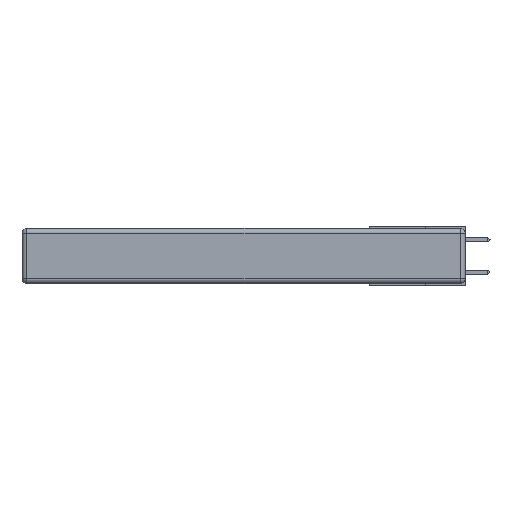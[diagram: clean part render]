
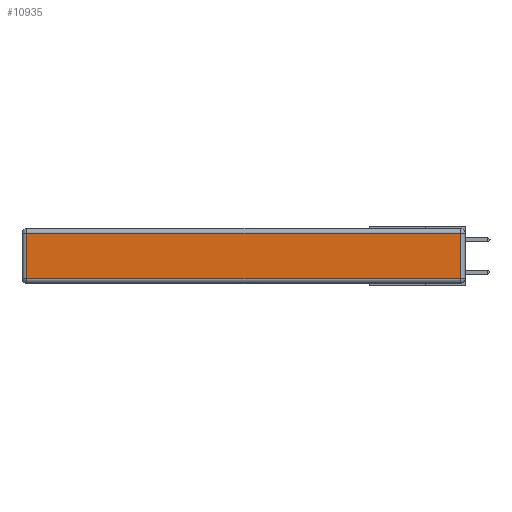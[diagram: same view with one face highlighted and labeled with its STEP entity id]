
A CAD part, left-side view. The second image highlights one B-rep face of the part: STEP entity #10935.
In plain terms, the highlighted planar face has unit normal (-1, 0, 0).
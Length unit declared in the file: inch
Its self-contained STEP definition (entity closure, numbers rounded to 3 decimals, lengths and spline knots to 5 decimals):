
#29 = CARTESIAN_POINT ( 'NONE',  ( 0., 2.72, -0.343 ) ) ;
#61 = VECTOR ( 'NONE', #6538, 39.37008 ) ;
#242 = VECTOR ( 'NONE', #2685, 39.37008 ) ;
#445 = ORIENTED_EDGE ( 'NONE', *, *, #8356, .T. ) ;
#621 = DIRECTION ( 'NONE',  ( 0., 1., 0. ) ) ;
#753 = VERTEX_POINT ( 'NONE', #1534 ) ;
#813 = EDGE_LOOP ( 'NONE', ( #6184, #445, #2058, #11182 ) ) ;
#819 = CARTESIAN_POINT ( 'NONE',  ( 0., 0.03, -0.03 ) ) ;
#1044 = CARTESIAN_POINT ( 'NONE',  ( 0., 0.03, -0.313 ) ) ;
#1534 = CARTESIAN_POINT ( 'NONE',  ( 0., 2.72, -0.313 ) ) ;
#2058 = ORIENTED_EDGE ( 'NONE', *, *, #11726, .T. ) ;
#2646 = DIRECTION ( 'NONE',  ( 0., 0., 1. ) ) ;
#2685 = DIRECTION ( 'NONE',  ( 0., 0., -1. ) ) ;
#2875 = LINE ( 'NONE', #6460, #61 ) ;
#3518 = CARTESIAN_POINT ( 'NONE',  ( 0., 0., -0.343 ) ) ;
#3528 = VERTEX_POINT ( 'NONE', #1044 ) ;
#3623 = VECTOR ( 'NONE', #10180, 39.37008 ) ;
#3630 = AXIS2_PLACEMENT_3D ( 'NONE', #3518, #8353, #2646 ) ;
#3816 = CARTESIAN_POINT ( 'NONE',  ( 0., 0., -0.313 ) ) ;
#5025 = LINE ( 'NONE', #9230, #7814 ) ;
#6184 = ORIENTED_EDGE ( 'NONE', *, *, #6351, .T. ) ;
#6336 = EDGE_CURVE ( 'NONE', #11303, #753, #6407, .T. ) ;
#6351 = EDGE_CURVE ( 'NONE', #753, #3528, #11774, .T. ) ;
#6407 = LINE ( 'NONE', #29, #242 ) ;
#6460 = CARTESIAN_POINT ( 'NONE',  ( 0., 0.03, -0.343 ) ) ;
#6538 = DIRECTION ( 'NONE',  ( 0., 0., 1. ) ) ;
#7560 = FACE_OUTER_BOUND ( 'NONE', #813, .T. ) ;
#7814 = VECTOR ( 'NONE', #621, 39.37008 ) ;
#8353 = DIRECTION ( 'NONE',  ( -1., 0., 0. ) ) ;
#8356 = EDGE_CURVE ( 'NONE', #3528, #9062, #2875, .T. ) ;
#8795 = CARTESIAN_POINT ( 'NONE',  ( 0., 2.72, -0.03 ) ) ;
#9062 = VERTEX_POINT ( 'NONE', #819 ) ;
#9230 = CARTESIAN_POINT ( 'NONE',  ( 0., 2.75, -0.03 ) ) ;
#10180 = DIRECTION ( 'NONE',  ( 0., -1., 0. ) ) ;
#10935 = ADVANCED_FACE ( 'NONE', ( #7560 ), #10983, .T. ) ;
#10983 = PLANE ( 'NONE',  #3630 ) ;
#11182 = ORIENTED_EDGE ( 'NONE', *, *, #6336, .T. ) ;
#11303 = VERTEX_POINT ( 'NONE', #8795 ) ;
#11726 = EDGE_CURVE ( 'NONE', #9062, #11303, #5025, .T. ) ;
#11774 = LINE ( 'NONE', #3816, #3623 ) ;
